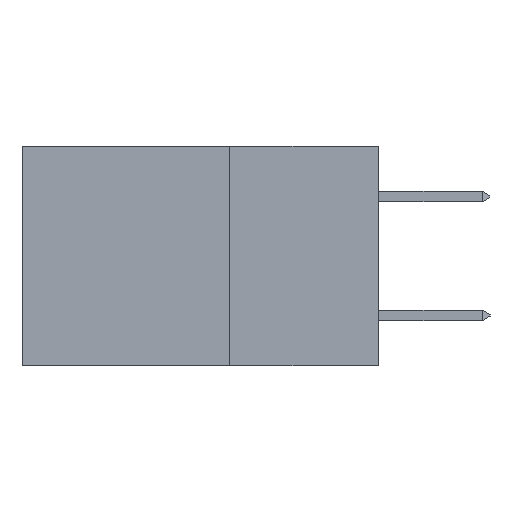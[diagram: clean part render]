
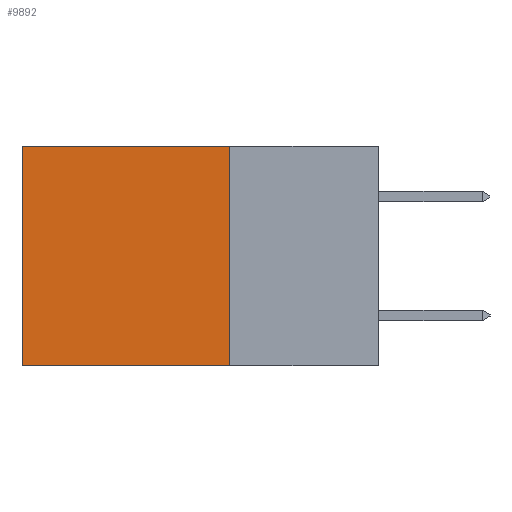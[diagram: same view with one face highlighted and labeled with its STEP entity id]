
A CAD part, left-side view. The second image highlights one B-rep face of the part: STEP entity #9892.
In plain terms, the highlighted planar face has unit normal (-1, 0, 0).
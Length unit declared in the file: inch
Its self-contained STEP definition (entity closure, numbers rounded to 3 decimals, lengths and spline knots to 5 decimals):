
#1679 = DIRECTION ( 'NONE',  ( 0., 1., 0. ) ) ;
#1796 = CARTESIAN_POINT ( 'NONE',  ( 0.2615, 0.25, -0.37 ) ) ;
#1954 = VECTOR ( 'NONE', #7981, 39.37008 ) ;
#2576 = DIRECTION ( 'NONE',  ( 0., 0., -1. ) ) ;
#2581 = DIRECTION ( 'NONE',  ( 1., 0., 0. ) ) ;
#2599 = CARTESIAN_POINT ( 'NONE',  ( 0.2615, 0.25, -0.37 ) ) ;
#2622 = PLANE ( 'NONE',  #11971 ) ;
#2983 = EDGE_CURVE ( 'NONE', #9805, #6014, #5678, .T. ) ;
#3074 = DIRECTION ( 'NONE',  ( 0., 0., -1. ) ) ;
#3333 = CARTESIAN_POINT ( 'NONE',  ( 0.2615, 0.25, 0. ) ) ;
#3412 = LINE ( 'NONE', #1796, #15575 ) ;
#3822 = EDGE_CURVE ( 'NONE', #11988, #6873, #13907, .T. ) ;
#4106 = VECTOR ( 'NONE', #1679, 39.37008 ) ;
#4822 = DIRECTION ( 'NONE',  ( 0., 0., -1. ) ) ;
#5678 = LINE ( 'NONE', #8433, #1954 ) ;
#6014 = VERTEX_POINT ( 'NONE', #7657 ) ;
#6614 = CARTESIAN_POINT ( 'NONE',  ( 0.2615, 0.6, -0.37 ) ) ;
#6744 = CARTESIAN_POINT ( 'NONE',  ( 0.2615, 0.25, -0.37 ) ) ;
#6873 = VERTEX_POINT ( 'NONE', #6614 ) ;
#7431 = CARTESIAN_POINT ( 'NONE',  ( 0.2615, 0.25, -0.37 ) ) ;
#7657 = CARTESIAN_POINT ( 'NONE',  ( 0.2615, 0.6, 0. ) ) ;
#7981 = DIRECTION ( 'NONE',  ( 0., 1., 0. ) ) ;
#8128 = ORIENTED_EDGE ( 'NONE', *, *, #3822, .F. ) ;
#8433 = CARTESIAN_POINT ( 'NONE',  ( 0.2615, 0.25, 0. ) ) ;
#8475 = LINE ( 'NONE', #12924, #14552 ) ;
#9102 = ORIENTED_EDGE ( 'NONE', *, *, #14380, .T. ) ;
#9805 = VERTEX_POINT ( 'NONE', #3333 ) ;
#9892 = ADVANCED_FACE ( 'NONE', ( #14017 ), #2622, .F. ) ;
#11320 = EDGE_CURVE ( 'NONE', #9805, #11988, #3412, .T. ) ;
#11971 = AXIS2_PLACEMENT_3D ( 'NONE', #2599, #2581, #2576 ) ;
#11988 = VERTEX_POINT ( 'NONE', #7431 ) ;
#12924 = CARTESIAN_POINT ( 'NONE',  ( 0.2615, 0.6, -0.37 ) ) ;
#13907 = LINE ( 'NONE', #6744, #4106 ) ;
#14017 = FACE_OUTER_BOUND ( 'NONE', #14687, .T. ) ;
#14380 = EDGE_CURVE ( 'NONE', #6014, #6873, #8475, .T. ) ;
#14552 = VECTOR ( 'NONE', #3074, 39.37008 ) ;
#14687 = EDGE_LOOP ( 'NONE', ( #9102, #8128, #15141, #14993 ) ) ;
#14993 = ORIENTED_EDGE ( 'NONE', *, *, #2983, .T. ) ;
#15141 = ORIENTED_EDGE ( 'NONE', *, *, #11320, .F. ) ;
#15575 = VECTOR ( 'NONE', #4822, 39.37008 ) ;
